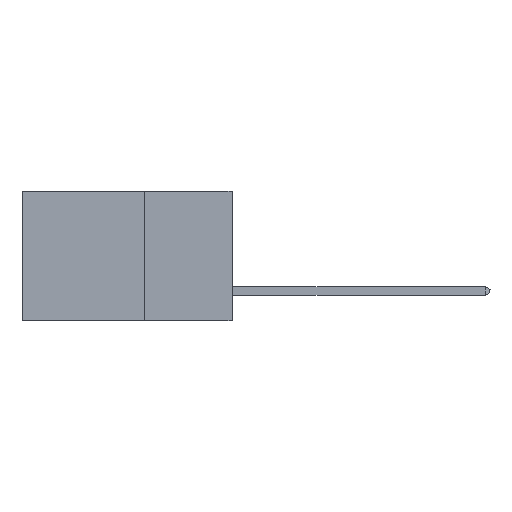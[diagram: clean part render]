
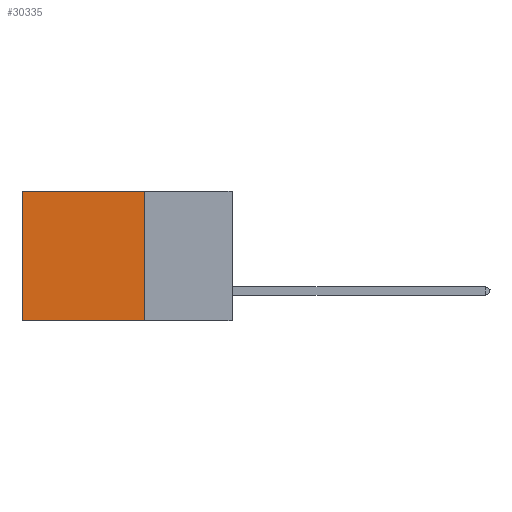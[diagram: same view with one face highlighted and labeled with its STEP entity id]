
A CAD part, left-side view. The second image highlights one B-rep face of the part: STEP entity #30335.
In plain terms, the highlighted planar face has unit normal (-1, 0, 0).
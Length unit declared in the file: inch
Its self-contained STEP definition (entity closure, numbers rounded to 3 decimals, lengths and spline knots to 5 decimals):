
#338 = CARTESIAN_POINT ( 'NONE',  ( 0.2875, 0.25, -0.37 ) ) ;
#1310 = VERTEX_POINT ( 'NONE', #23115 ) ;
#5801 = LINE ( 'NONE', #11179, #13365 ) ;
#9068 = LINE ( 'NONE', #21566, #21270 ) ;
#9335 = CARTESIAN_POINT ( 'NONE',  ( 0.2875, 0.6, 0. ) ) ;
#10067 = EDGE_CURVE ( 'NONE', #28107, #26370, #9068, .T. ) ;
#10885 = DIRECTION ( 'NONE',  ( 0., 0., -1. ) ) ;
#11179 = CARTESIAN_POINT ( 'NONE',  ( 0.2875, 0.25, -0.37 ) ) ;
#12320 = EDGE_CURVE ( 'NONE', #1310, #25130, #30144, .T. ) ;
#12609 = DIRECTION ( 'NONE',  ( 0., 0., -1. ) ) ;
#13187 = DIRECTION ( 'NONE',  ( 1., 0., 0. ) ) ;
#13365 = VECTOR ( 'NONE', #25707, 39.37008 ) ;
#13396 = VECTOR ( 'NONE', #12609, 39.37008 ) ;
#15471 = PLANE ( 'NONE',  #28182 ) ;
#16171 = DIRECTION ( 'NONE',  ( 0., 1., 0. ) ) ;
#17280 = EDGE_CURVE ( 'NONE', #28107, #1310, #26901, .T. ) ;
#17400 = EDGE_LOOP ( 'NONE', ( #25850, #23554, #28040, #30986 ) ) ;
#18554 = EDGE_CURVE ( 'NONE', #26370, #25130, #5801, .T. ) ;
#20432 = CARTESIAN_POINT ( 'NONE',  ( 0.2875, 0.25, 0. ) ) ;
#20865 = CARTESIAN_POINT ( 'NONE',  ( 0.2875, 0.25, 0. ) ) ;
#21270 = VECTOR ( 'NONE', #21810, 39.37008 ) ;
#21566 = CARTESIAN_POINT ( 'NONE',  ( 0.2875, 0.25, 0. ) ) ;
#21810 = DIRECTION ( 'NONE',  ( 0., 0., -1. ) ) ;
#22607 = CARTESIAN_POINT ( 'NONE',  ( 0.2875, 0.6, -0.37 ) ) ;
#22759 = CARTESIAN_POINT ( 'NONE',  ( 0.2875, 0.25, 0. ) ) ;
#23115 = CARTESIAN_POINT ( 'NONE',  ( 0.2875, 0.6, 0. ) ) ;
#23554 = ORIENTED_EDGE ( 'NONE', *, *, #18554, .F. ) ;
#25130 = VERTEX_POINT ( 'NONE', #22607 ) ;
#25707 = DIRECTION ( 'NONE',  ( 0., 1., 0. ) ) ;
#25850 = ORIENTED_EDGE ( 'NONE', *, *, #12320, .T. ) ;
#26169 = VECTOR ( 'NONE', #16171, 39.37008 ) ;
#26370 = VERTEX_POINT ( 'NONE', #338 ) ;
#26901 = LINE ( 'NONE', #20865, #26169 ) ;
#28040 = ORIENTED_EDGE ( 'NONE', *, *, #10067, .F. ) ;
#28107 = VERTEX_POINT ( 'NONE', #22759 ) ;
#28182 = AXIS2_PLACEMENT_3D ( 'NONE', #20432, #13187, #10885 ) ;
#29889 = FACE_OUTER_BOUND ( 'NONE', #17400, .T. ) ;
#30144 = LINE ( 'NONE', #9335, #13396 ) ;
#30335 = ADVANCED_FACE ( 'NONE', ( #29889 ), #15471, .F. ) ;
#30986 = ORIENTED_EDGE ( 'NONE', *, *, #17280, .T. ) ;
